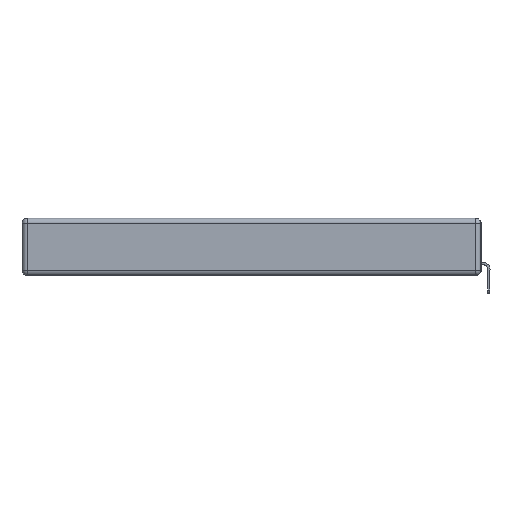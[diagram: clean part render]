
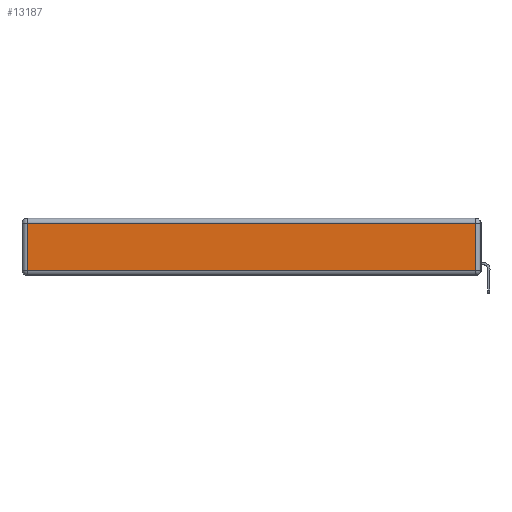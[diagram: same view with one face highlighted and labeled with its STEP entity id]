
A CAD part, left-side view. The second image highlights one B-rep face of the part: STEP entity #13187.
In plain terms, the highlighted planar face has unit normal (-1, 0, 0).
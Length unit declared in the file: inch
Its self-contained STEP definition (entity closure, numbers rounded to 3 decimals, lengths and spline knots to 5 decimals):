
#188 = CARTESIAN_POINT ( 'NONE',  ( 0., 2.72, -0.03 ) ) ;
#869 = ORIENTED_EDGE ( 'NONE', *, *, #9974, .T. ) ;
#1464 = CARTESIAN_POINT ( 'NONE',  ( 0., 0.03, -0.03 ) ) ;
#1695 = CARTESIAN_POINT ( 'NONE',  ( 0., 0., -0.343 ) ) ;
#1801 = VERTEX_POINT ( 'NONE', #1464 ) ;
#2166 = VERTEX_POINT ( 'NONE', #188 ) ;
#2658 = LINE ( 'NONE', #6402, #10861 ) ;
#2737 = DIRECTION ( 'NONE',  ( -1., 0., 0. ) ) ;
#3368 = DIRECTION ( 'NONE',  ( 0., 0., 1. ) ) ;
#5161 = DIRECTION ( 'NONE',  ( 0., 1., 0. ) ) ;
#5626 = VECTOR ( 'NONE', #11765, 39.37008 ) ;
#6402 = CARTESIAN_POINT ( 'NONE',  ( 0., 2.75, -0.03 ) ) ;
#6980 = LINE ( 'NONE', #7759, #7297 ) ;
#7297 = VECTOR ( 'NONE', #3368, 39.37008 ) ;
#7663 = ORIENTED_EDGE ( 'NONE', *, *, #10204, .T. ) ;
#7676 = FACE_OUTER_BOUND ( 'NONE', #7697, .T. ) ;
#7697 = EDGE_LOOP ( 'NONE', ( #9849, #7663, #11657, #869 ) ) ;
#7759 = CARTESIAN_POINT ( 'NONE',  ( 0., 0.03, -0.343 ) ) ;
#7981 = LINE ( 'NONE', #11670, #13524 ) ;
#8152 = EDGE_CURVE ( 'NONE', #1801, #2166, #2658, .T. ) ;
#8538 = CARTESIAN_POINT ( 'NONE',  ( 0., 2.72, -0.343 ) ) ;
#8622 = DIRECTION ( 'NONE',  ( 0., -1., 0. ) ) ;
#9003 = VERTEX_POINT ( 'NONE', #13041 ) ;
#9849 = ORIENTED_EDGE ( 'NONE', *, *, #10010, .T. ) ;
#9974 = EDGE_CURVE ( 'NONE', #2166, #9003, #13855, .T. ) ;
#10010 = EDGE_CURVE ( 'NONE', #9003, #12615, #7981, .T. ) ;
#10204 = EDGE_CURVE ( 'NONE', #12615, #1801, #6980, .T. ) ;
#10861 = VECTOR ( 'NONE', #5161, 39.37008 ) ;
#11235 = CARTESIAN_POINT ( 'NONE',  ( 0., 0.03, -0.313 ) ) ;
#11657 = ORIENTED_EDGE ( 'NONE', *, *, #8152, .T. ) ;
#11670 = CARTESIAN_POINT ( 'NONE',  ( 0., 0., -0.313 ) ) ;
#11765 = DIRECTION ( 'NONE',  ( 0., 0., -1. ) ) ;
#12498 = PLANE ( 'NONE',  #13300 ) ;
#12615 = VERTEX_POINT ( 'NONE', #11235 ) ;
#13041 = CARTESIAN_POINT ( 'NONE',  ( 0., 2.72, -0.313 ) ) ;
#13187 = ADVANCED_FACE ( 'NONE', ( #7676 ), #12498, .T. ) ;
#13300 = AXIS2_PLACEMENT_3D ( 'NONE', #1695, #2737, #13590 ) ;
#13524 = VECTOR ( 'NONE', #8622, 39.37008 ) ;
#13590 = DIRECTION ( 'NONE',  ( 0., 0., 1. ) ) ;
#13855 = LINE ( 'NONE', #8538, #5626 ) ;
